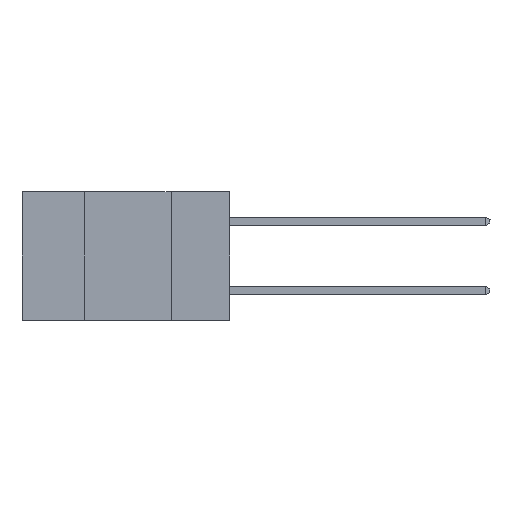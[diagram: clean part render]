
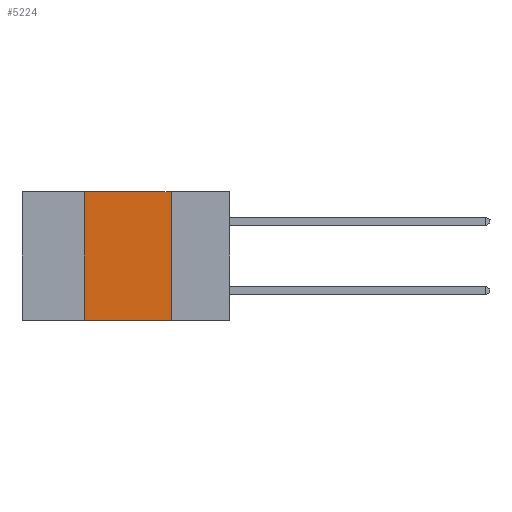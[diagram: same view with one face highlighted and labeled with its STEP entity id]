
A CAD part, left-side view. The second image highlights one B-rep face of the part: STEP entity #5224.
In plain terms, the highlighted planar face has unit normal (-1, 0, 0).
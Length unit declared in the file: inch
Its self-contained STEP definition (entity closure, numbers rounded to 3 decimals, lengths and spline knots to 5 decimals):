
#41 = VERTEX_POINT ( 'NONE', #7786 ) ;
#91 = CARTESIAN_POINT ( 'NONE',  ( 0., 0.6, 0. ) ) ;
#150 = ORIENTED_EDGE ( 'NONE', *, *, #11273, .F. ) ;
#768 = LINE ( 'NONE', #2597, #1096 ) ;
#1096 = VECTOR ( 'NONE', #5529, 39.37008 ) ;
#1408 = CARTESIAN_POINT ( 'NONE',  ( 0., 0.17, -0.37 ) ) ;
#1551 = CARTESIAN_POINT ( 'NONE',  ( 0., 0.42, -0.37 ) ) ;
#1964 = CARTESIAN_POINT ( 'NONE',  ( 0., 0.17, 0. ) ) ;
#2180 = VECTOR ( 'NONE', #9422, 39.37008 ) ;
#2225 = VERTEX_POINT ( 'NONE', #1408 ) ;
#2442 = LINE ( 'NONE', #9701, #4359 ) ;
#2501 = EDGE_CURVE ( 'NONE', #41, #8468, #8222, .T. ) ;
#2597 = CARTESIAN_POINT ( 'NONE',  ( 0., 0.17, -0.37 ) ) ;
#2905 = ORIENTED_EDGE ( 'NONE', *, *, #10369, .F. ) ;
#3329 = AXIS2_PLACEMENT_3D ( 'NONE', #11396, #8815, #5929 ) ;
#3883 = ORIENTED_EDGE ( 'NONE', *, *, #11747, .T. ) ;
#4359 = VECTOR ( 'NONE', #8800, 39.37008 ) ;
#4930 = VECTOR ( 'NONE', #11743, 39.37008 ) ;
#5224 = ADVANCED_FACE ( 'NONE', ( #7857 ), #6047, .F. ) ;
#5461 = ORIENTED_EDGE ( 'NONE', *, *, #2501, .F. ) ;
#5529 = DIRECTION ( 'NONE',  ( 0., 0., -1. ) ) ;
#5929 = DIRECTION ( 'NONE',  ( 0., 0., -1. ) ) ;
#6047 = PLANE ( 'NONE',  #3329 ) ;
#6782 = VERTEX_POINT ( 'NONE', #11211 ) ;
#7786 = CARTESIAN_POINT ( 'NONE',  ( 0., 0.42, 0. ) ) ;
#7857 = FACE_OUTER_BOUND ( 'NONE', #10457, .T. ) ;
#8222 = LINE ( 'NONE', #91, #2180 ) ;
#8468 = VERTEX_POINT ( 'NONE', #1964 ) ;
#8800 = DIRECTION ( 'NONE',  ( 0., -1., 0. ) ) ;
#8815 = DIRECTION ( 'NONE',  ( 1., 0., 0. ) ) ;
#9422 = DIRECTION ( 'NONE',  ( 0., -1., 0. ) ) ;
#9701 = CARTESIAN_POINT ( 'NONE',  ( 0., 0.6, -0.37 ) ) ;
#9712 = LINE ( 'NONE', #1551, #4930 ) ;
#10369 = EDGE_CURVE ( 'NONE', #8468, #2225, #768, .T. ) ;
#10457 = EDGE_LOOP ( 'NONE', ( #2905, #5461, #150, #3883 ) ) ;
#11211 = CARTESIAN_POINT ( 'NONE',  ( 0., 0.42, -0.37 ) ) ;
#11273 = EDGE_CURVE ( 'NONE', #6782, #41, #9712, .T. ) ;
#11396 = CARTESIAN_POINT ( 'NONE',  ( 0., 0.6, 0. ) ) ;
#11743 = DIRECTION ( 'NONE',  ( 0., 0., 1. ) ) ;
#11747 = EDGE_CURVE ( 'NONE', #6782, #2225, #2442, .T. ) ;
